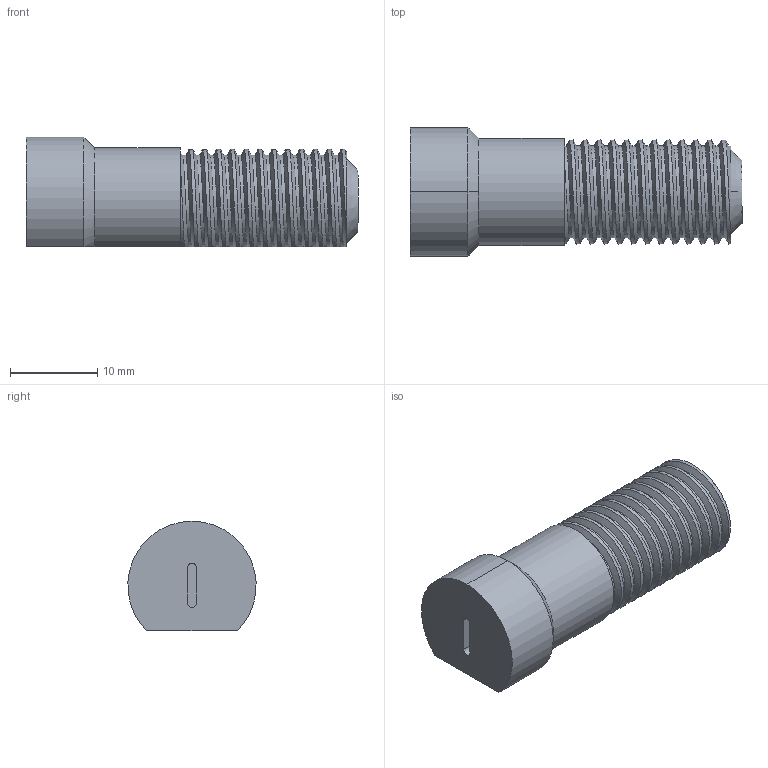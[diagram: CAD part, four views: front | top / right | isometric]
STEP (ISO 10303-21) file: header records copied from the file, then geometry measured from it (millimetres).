
FILE_DESCRIPTION (( 'STEP AP203' ), '1' );
FILE_NAME ('AF-WF-LR-PRT-005-STEP.STEP', '2020-07-21T18:17:18', ( '' ), ( '' ), 'SwSTEP 2.0', 'SolidWorks 2018', '' );
FILE_SCHEMA (( 'CONFIG_CONTROL_DESIGN' ));
Length unit declared in the file: inch
Products named in the file (1): AF-WF-LR-PRT-005-STEP
Bounding box: 38.1 x 14.71 x 12.57 mm (x, y, z)
Volume: 4253.2 mm3; surface area: 2039.9 mm2
Topology: 1 solids, 1 shells, 71 faces, 200 edges, 133 vertices
Faces by surface type: bspline 40, cylinder 19, plane 8, cone 4
Entity records: 23418 total; most frequent: CARTESIAN_POINT 21987, ORIENTED_EDGE 400, EDGE_CURVE 200, DIRECTION 147, VERTEX_POINT 133, EDGE_LOOP 73, FACE_OUTER_BOUND 71, ADVANCED_FACE 71
